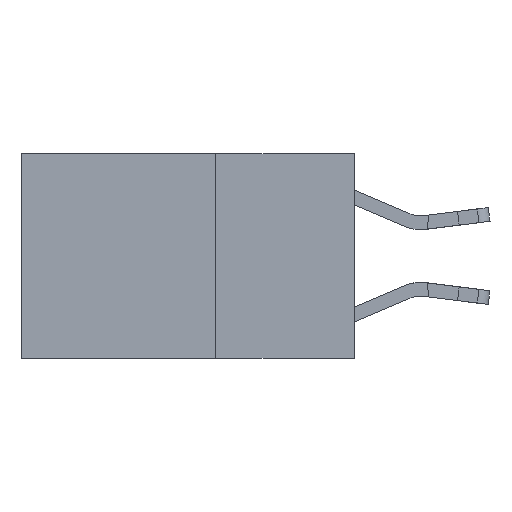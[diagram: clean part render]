
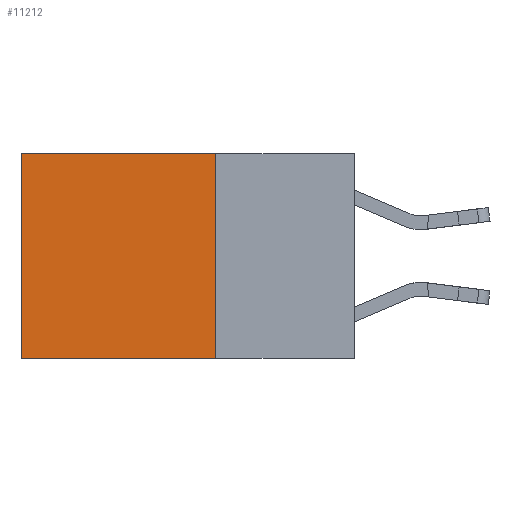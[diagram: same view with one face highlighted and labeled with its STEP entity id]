
A CAD part, left-side view. The second image highlights one B-rep face of the part: STEP entity #11212.
In plain terms, the highlighted planar face has unit normal (-1, 0, 0).
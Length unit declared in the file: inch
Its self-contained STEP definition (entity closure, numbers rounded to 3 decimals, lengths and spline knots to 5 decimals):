
#414 = VERTEX_POINT ( 'NONE', #12180 ) ;
#1144 = ORIENTED_EDGE ( 'NONE', *, *, #15762, .F. ) ;
#1856 = LINE ( 'NONE', #13872, #10135 ) ;
#1898 = ORIENTED_EDGE ( 'NONE', *, *, #12143, .T. ) ;
#2264 = EDGE_CURVE ( 'NONE', #7421, #9557, #13684, .T. ) ;
#2265 = LINE ( 'NONE', #8511, #15558 ) ;
#2567 = DIRECTION ( 'NONE',  ( 0., 1., 0. ) ) ;
#2679 = DIRECTION ( 'NONE',  ( 0., 1., 0. ) ) ;
#2768 = VECTOR ( 'NONE', #2679, 39.37008 ) ;
#4477 = VECTOR ( 'NONE', #9788, 39.37008 ) ;
#6272 = VERTEX_POINT ( 'NONE', #6733 ) ;
#6733 = CARTESIAN_POINT ( 'NONE',  ( 0.2625, 0.6, 0. ) ) ;
#7276 = CARTESIAN_POINT ( 'NONE',  ( 0.2625, 0.25, 0. ) ) ;
#7421 = VERTEX_POINT ( 'NONE', #16275 ) ;
#7640 = CARTESIAN_POINT ( 'NONE',  ( 0.2625, 0.6, -0.37 ) ) ;
#7966 = DIRECTION ( 'NONE',  ( 0., 0., -1. ) ) ;
#8511 = CARTESIAN_POINT ( 'NONE',  ( 0.2625, 0.6, 0. ) ) ;
#9227 = PLANE ( 'NONE',  #13663 ) ;
#9285 = ORIENTED_EDGE ( 'NONE', *, *, #12187, .T. ) ;
#9557 = VERTEX_POINT ( 'NONE', #7640 ) ;
#9788 = DIRECTION ( 'NONE',  ( 0., 0., -1. ) ) ;
#10135 = VECTOR ( 'NONE', #2567, 39.37008 ) ;
#10156 = LINE ( 'NONE', #7276, #4477 ) ;
#11018 = DIRECTION ( 'NONE',  ( 0., 0., -1. ) ) ;
#11212 = ADVANCED_FACE ( 'NONE', ( #13406 ), #9227, .F. ) ;
#11561 = DIRECTION ( 'NONE',  ( 1., 0., 0. ) ) ;
#11785 = CARTESIAN_POINT ( 'NONE',  ( 0.2625, 0.25, 0. ) ) ;
#12143 = EDGE_CURVE ( 'NONE', #6272, #9557, #2265, .T. ) ;
#12180 = CARTESIAN_POINT ( 'NONE',  ( 0.2625, 0.25, 0. ) ) ;
#12187 = EDGE_CURVE ( 'NONE', #414, #6272, #1856, .T. ) ;
#12885 = EDGE_LOOP ( 'NONE', ( #1898, #13336, #1144, #9285 ) ) ;
#13336 = ORIENTED_EDGE ( 'NONE', *, *, #2264, .F. ) ;
#13406 = FACE_OUTER_BOUND ( 'NONE', #12885, .T. ) ;
#13663 = AXIS2_PLACEMENT_3D ( 'NONE', #11785, #11561, #7966 ) ;
#13684 = LINE ( 'NONE', #16399, #2768 ) ;
#13872 = CARTESIAN_POINT ( 'NONE',  ( 0.2625, 0.25, 0. ) ) ;
#15558 = VECTOR ( 'NONE', #11018, 39.37008 ) ;
#15762 = EDGE_CURVE ( 'NONE', #414, #7421, #10156, .T. ) ;
#16275 = CARTESIAN_POINT ( 'NONE',  ( 0.2625, 0.25, -0.37 ) ) ;
#16399 = CARTESIAN_POINT ( 'NONE',  ( 0.2625, 0.25, -0.37 ) ) ;
